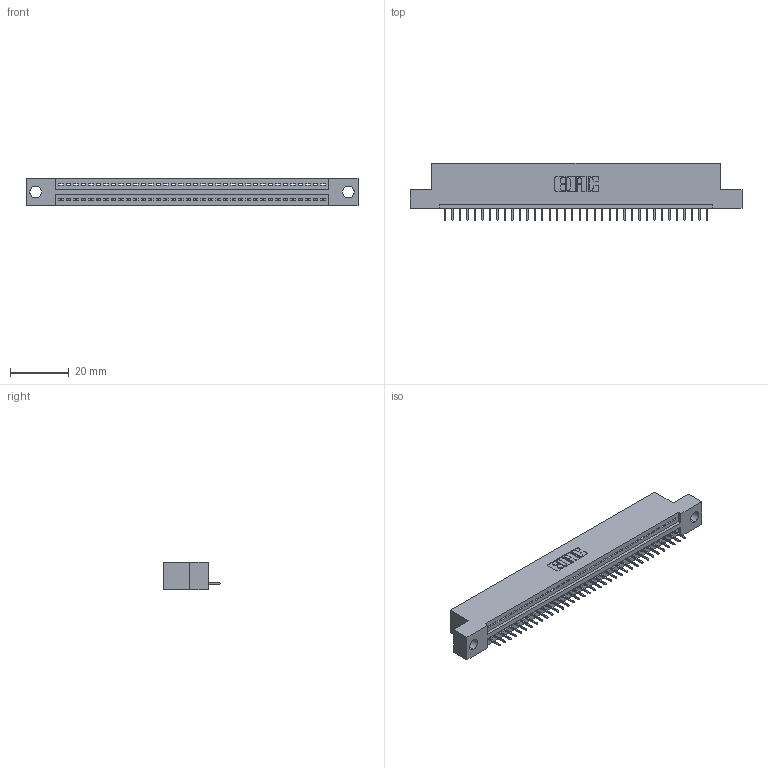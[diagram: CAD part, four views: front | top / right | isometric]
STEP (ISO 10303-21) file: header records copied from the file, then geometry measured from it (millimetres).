
FILE_DESCRIPTION (( 'STEP AP203' ), '1' );
FILE_NAME ('345-036-524-104.STEP', '2019-10-07T22:52:38', ( '' ), ( '' ), 'SwSTEP 2.0', 'SolidWorks 2016', '' );
FILE_SCHEMA (( 'CONFIG_CONTROL_DESIGN' ));
Length unit declared in the file: inch
Products named in the file (3): 345-036-524-104; 345-292-001_345-293-124; 345 Part_Flush Mounting Lugs - 0.156 Dia-TH
Assembly tree (37 placements, depth 2):
  345-036-524-104
    345 Part_Flush Mounting Lugs - 0.156 Dia-TH
    345-292-001_345-293-124  x36
Bounding box: 112.65 x 19.35 x 9.4 mm (x, y, z)
Volume: 10420.3 mm3; surface area: 13120.2 mm2
Topology: 37 solids, 37 shells, 2358 faces, 6821 edges, 4402 vertices
Faces by surface type: plane 1736, cylinder 622
Entity records: 27979 total; most frequent: CARTESIAN_POINT 4852, ORIENTED_EDGE 4822, DIRECTION 4247, EDGE_CURVE 2411, LINE 2139, VECTOR 2139, VERTEX_POINT 1602, AXIS2_PLACEMENT_3D 1054
